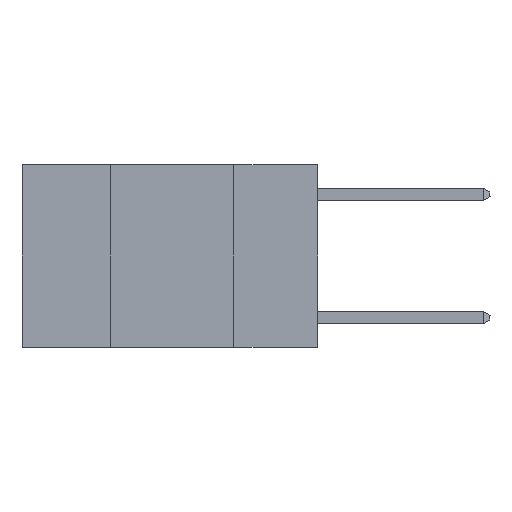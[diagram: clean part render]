
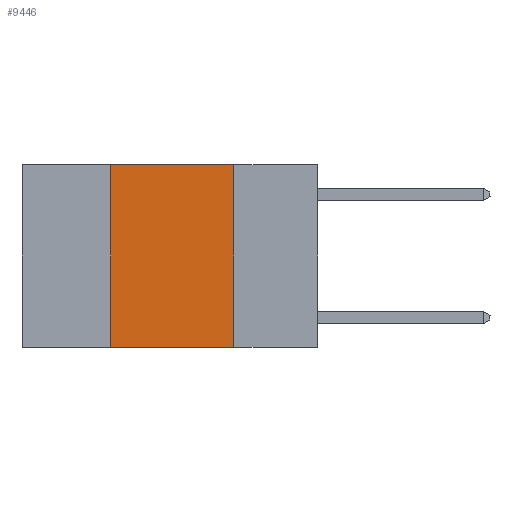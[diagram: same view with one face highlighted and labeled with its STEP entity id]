
A CAD part, left-side view. The second image highlights one B-rep face of the part: STEP entity #9446.
In plain terms, the highlighted planar face has unit normal (-1, 0, 0).
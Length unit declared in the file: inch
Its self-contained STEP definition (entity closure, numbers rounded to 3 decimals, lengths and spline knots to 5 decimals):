
#713 = CARTESIAN_POINT ( 'NONE',  ( 0., 0.17, 0. ) ) ;
#1240 = CARTESIAN_POINT ( 'NONE',  ( 0., 0.42, 0. ) ) ;
#2764 = FACE_OUTER_BOUND ( 'NONE', #5325, .T. ) ;
#3049 = PLANE ( 'NONE',  #4033 ) ;
#3228 = DIRECTION ( 'NONE',  ( 0., -1., 0. ) ) ;
#3983 = EDGE_CURVE ( 'NONE', #22972, #15999, #25597, .T. ) ;
#4033 = AXIS2_PLACEMENT_3D ( 'NONE', #18072, #4789, #16054 ) ;
#4081 = CARTESIAN_POINT ( 'NONE',  ( 0., 0.17, -0.37 ) ) ;
#4576 = EDGE_CURVE ( 'NONE', #7835, #22972, #15687, .T. ) ;
#4789 = DIRECTION ( 'NONE',  ( 1., 0., 0. ) ) ;
#5325 = EDGE_LOOP ( 'NONE', ( #7936, #19393, #27053, #14730 ) ) ;
#6334 = CARTESIAN_POINT ( 'NONE',  ( 0., 0.42, 0. ) ) ;
#6801 = DIRECTION ( 'NONE',  ( 0., 0., -1. ) ) ;
#7219 = VECTOR ( 'NONE', #6801, 39.37008 ) ;
#7835 = VERTEX_POINT ( 'NONE', #6334 ) ;
#7936 = ORIENTED_EDGE ( 'NONE', *, *, #3983, .F. ) ;
#8359 = CARTESIAN_POINT ( 'NONE',  ( 0., 0.6, 0. ) ) ;
#9123 = VERTEX_POINT ( 'NONE', #23152 ) ;
#9446 = ADVANCED_FACE ( 'NONE', ( #2764 ), #3049, .F. ) ;
#10071 = DIRECTION ( 'NONE',  ( 0., 0., 1. ) ) ;
#12114 = LINE ( 'NONE', #1240, #23202 ) ;
#14730 = ORIENTED_EDGE ( 'NONE', *, *, #19545, .T. ) ;
#15687 = LINE ( 'NONE', #8359, #25441 ) ;
#15999 = VERTEX_POINT ( 'NONE', #4081 ) ;
#16054 = DIRECTION ( 'NONE',  ( 0., 0., -1. ) ) ;
#18072 = CARTESIAN_POINT ( 'NONE',  ( 0., 0.6, 0. ) ) ;
#19393 = ORIENTED_EDGE ( 'NONE', *, *, #4576, .F. ) ;
#19545 = EDGE_CURVE ( 'NONE', #9123, #15999, #25476, .T. ) ;
#22972 = VERTEX_POINT ( 'NONE', #713 ) ;
#23018 = CARTESIAN_POINT ( 'NONE',  ( 0., 0.6, -0.37 ) ) ;
#23152 = CARTESIAN_POINT ( 'NONE',  ( 0., 0.42, -0.37 ) ) ;
#23202 = VECTOR ( 'NONE', #10071, 39.37008 ) ;
#25441 = VECTOR ( 'NONE', #26657, 39.37008 ) ;
#25476 = LINE ( 'NONE', #23018, #25498 ) ;
#25498 = VECTOR ( 'NONE', #3228, 39.37008 ) ;
#25597 = LINE ( 'NONE', #26587, #7219 ) ;
#26587 = CARTESIAN_POINT ( 'NONE',  ( 0., 0.17, 0. ) ) ;
#26657 = DIRECTION ( 'NONE',  ( 0., -1., 0. ) ) ;
#27053 = ORIENTED_EDGE ( 'NONE', *, *, #28067, .F. ) ;
#28067 = EDGE_CURVE ( 'NONE', #9123, #7835, #12114, .T. ) ;
